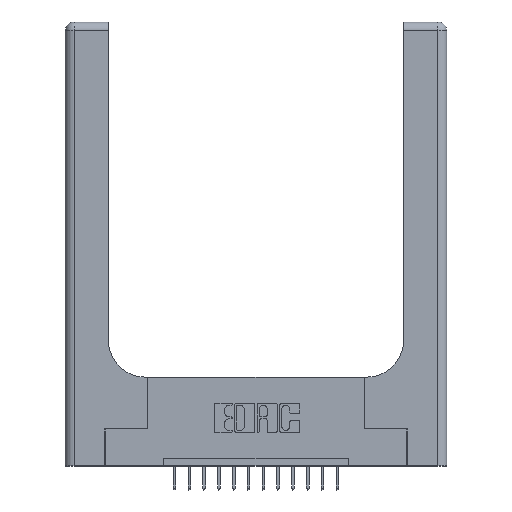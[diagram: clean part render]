
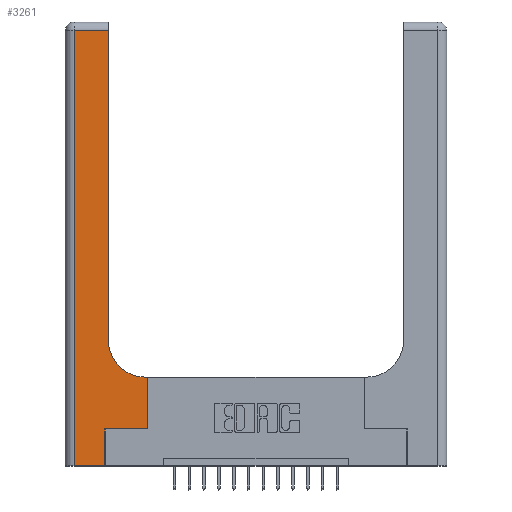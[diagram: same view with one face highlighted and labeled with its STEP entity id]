
A CAD part, top view. The second image highlights one B-rep face of the part: STEP entity #3261.
In plain terms, the highlighted planar face has unit normal (0, 0, 1).
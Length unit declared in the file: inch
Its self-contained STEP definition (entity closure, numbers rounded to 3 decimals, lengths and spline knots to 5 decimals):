
#696 = ORIENTED_EDGE ( 'NONE', *, *, #5143, .T. ) ;
#1784 = VECTOR ( 'NONE', #12385, 39.37008 ) ;
#2039 = CARTESIAN_POINT ( 'NONE',  ( 0.5415, 0.85, 0.37 ) ) ;
#2169 = CARTESIAN_POINT ( 'NONE',  ( 0.2915, 0.6, 0.37 ) ) ;
#2192 = DIRECTION ( 'NONE',  ( 0., 1., 0. ) ) ;
#2672 = VERTEX_POINT ( 'NONE', #12113 ) ;
#2764 = LINE ( 'NONE', #5634, #11132 ) ;
#2860 = DIRECTION ( 'NONE',  ( 0., -1., 0. ) ) ;
#2873 = CARTESIAN_POINT ( 'NONE',  ( 0.5585, 0.6, 0.37 ) ) ;
#2881 = ORIENTED_EDGE ( 'NONE', *, *, #8782, .T. ) ;
#3035 = CARTESIAN_POINT ( 'NONE',  ( 0.06, 3., 0.37 ) ) ;
#3261 = ADVANCED_FACE ( 'NONE', ( #14895 ), #6105, .F. ) ;
#3327 = LINE ( 'NONE', #9516, #1784 ) ;
#3738 = AXIS2_PLACEMENT_3D ( 'NONE', #4827, #18241, #17748 ) ;
#3750 = LINE ( 'NONE', #10135, #10337 ) ;
#4146 = VERTEX_POINT ( 'NONE', #2873 ) ;
#4154 = CARTESIAN_POINT ( 'NONE',  ( 0.06, 2.94, 0.37 ) ) ;
#4757 = VECTOR ( 'NONE', #18083, 39.37008 ) ;
#4827 = CARTESIAN_POINT ( 'NONE',  ( 0., 3., 0.37 ) ) ;
#4873 = DIRECTION ( 'NONE',  ( -1., 0., 0. ) ) ;
#4992 = VERTEX_POINT ( 'NONE', #4154 ) ;
#5143 = EDGE_CURVE ( 'NONE', #16495, #16221, #10296, .T. ) ;
#5190 = VECTOR ( 'NONE', #2192, 39.37008 ) ;
#5602 = ORIENTED_EDGE ( 'NONE', *, *, #6916, .T. ) ;
#5634 = CARTESIAN_POINT ( 'NONE',  ( 0.2915, 3., 0.37 ) ) ;
#5635 = ORIENTED_EDGE ( 'NONE', *, *, #9965, .T. ) ;
#5758 = CARTESIAN_POINT ( 'NONE',  ( 0.269, 0.25, 0.37 ) ) ;
#5817 = EDGE_CURVE ( 'NONE', #4992, #11446, #11824, .T. ) ;
#5872 = EDGE_CURVE ( 'NONE', #11446, #2672, #14705, .T. ) ;
#5890 = CARTESIAN_POINT ( 'NONE',  ( 0.5585, 0.25, 0.37 ) ) ;
#6034 = ORIENTED_EDGE ( 'NONE', *, *, #5817, .T. ) ;
#6066 = DIRECTION ( 'NONE',  ( 0., 1., 0. ) ) ;
#6105 = PLANE ( 'NONE',  #3738 ) ;
#6536 = VECTOR ( 'NONE', #2860, 39.37008 ) ;
#6660 = CARTESIAN_POINT ( 'NONE',  ( 0., 0., 0.37 ) ) ;
#6916 = EDGE_CURVE ( 'NONE', #2672, #11909, #16476, .T. ) ;
#7497 = VECTOR ( 'NONE', #4873, 39.37008 ) ;
#7806 = EDGE_LOOP ( 'NONE', ( #8874, #10061, #6034, #7828, #5602, #15420, #5635, #2881, #696 ) ) ;
#7828 = ORIENTED_EDGE ( 'NONE', *, *, #5872, .T. ) ;
#8778 = CARTESIAN_POINT ( 'NONE',  ( 0.2915, 0.85, 0.37 ) ) ;
#8782 = EDGE_CURVE ( 'NONE', #4146, #16495, #17935, .T. ) ;
#8874 = ORIENTED_EDGE ( 'NONE', *, *, #17247, .T. ) ;
#8891 = DIRECTION ( 'NONE',  ( 1., 0., 0. ) ) ;
#8902 = EDGE_CURVE ( 'NONE', #11036, #4992, #3327, .T. ) ;
#9414 = DIRECTION ( 'NONE',  ( 1., 0., 0. ) ) ;
#9516 = CARTESIAN_POINT ( 'NONE',  ( 0., 2.94, 0.37 ) ) ;
#9965 = EDGE_CURVE ( 'NONE', #13563, #4146, #3750, .T. ) ;
#10061 = ORIENTED_EDGE ( 'NONE', *, *, #8902, .T. ) ;
#10135 = CARTESIAN_POINT ( 'NONE',  ( 0.5585, 0.25, 0.37 ) ) ;
#10296 = CIRCLE ( 'NONE', #18327, 0.25 ) ;
#10337 = VECTOR ( 'NONE', #6066, 39.37008 ) ;
#11036 = VERTEX_POINT ( 'NONE', #11710 ) ;
#11132 = VECTOR ( 'NONE', #11357, 39.37008 ) ;
#11357 = DIRECTION ( 'NONE',  ( 0., 1., 0. ) ) ;
#11446 = VERTEX_POINT ( 'NONE', #17997 ) ;
#11710 = CARTESIAN_POINT ( 'NONE',  ( 0.2915, 2.94, 0.37 ) ) ;
#11824 = LINE ( 'NONE', #3035, #6536 ) ;
#11909 = VERTEX_POINT ( 'NONE', #5758 ) ;
#12113 = CARTESIAN_POINT ( 'NONE',  ( 0.269, 0., 0.37 ) ) ;
#12385 = DIRECTION ( 'NONE',  ( -1., 0., 0. ) ) ;
#12460 = CARTESIAN_POINT ( 'NONE',  ( 0.5415, 0.6, 0.37 ) ) ;
#13224 = CARTESIAN_POINT ( 'NONE',  ( 0.269, 0., 0.37 ) ) ;
#13563 = VERTEX_POINT ( 'NONE', #5890 ) ;
#14705 = LINE ( 'NONE', #6660, #17371 ) ;
#14895 = FACE_OUTER_BOUND ( 'NONE', #7806, .T. ) ;
#15340 = CARTESIAN_POINT ( 'NONE',  ( 0.269, 0.25, 0.37 ) ) ;
#15420 = ORIENTED_EDGE ( 'NONE', *, *, #17615, .T. ) ;
#16221 = VERTEX_POINT ( 'NONE', #8778 ) ;
#16476 = LINE ( 'NONE', #13224, #5190 ) ;
#16495 = VERTEX_POINT ( 'NONE', #12460 ) ;
#17134 = LINE ( 'NONE', #15340, #4757 ) ;
#17247 = EDGE_CURVE ( 'NONE', #16221, #11036, #2764, .T. ) ;
#17371 = VECTOR ( 'NONE', #9414, 39.37008 ) ;
#17587 = DIRECTION ( 'NONE',  ( 0., 0., -1. ) ) ;
#17615 = EDGE_CURVE ( 'NONE', #11909, #13563, #17134, .T. ) ;
#17748 = DIRECTION ( 'NONE',  ( -1., 0., 0. ) ) ;
#17935 = LINE ( 'NONE', #2169, #7497 ) ;
#17997 = CARTESIAN_POINT ( 'NONE',  ( 0.06, 0., 0.37 ) ) ;
#18083 = DIRECTION ( 'NONE',  ( 1., 0., 0. ) ) ;
#18241 = DIRECTION ( 'NONE',  ( 0., 0., -1. ) ) ;
#18327 = AXIS2_PLACEMENT_3D ( 'NONE', #2039, #17587, #8891 ) ;
